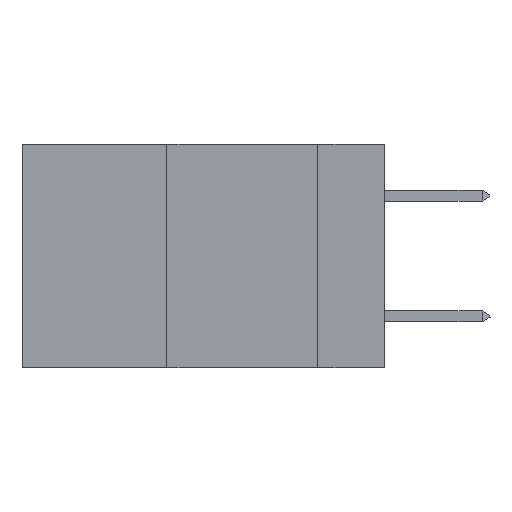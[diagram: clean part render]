
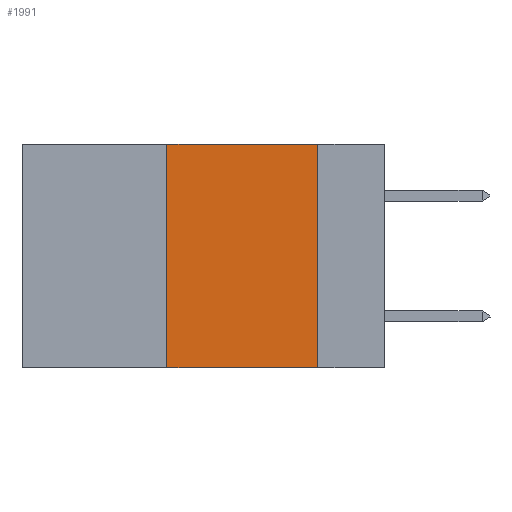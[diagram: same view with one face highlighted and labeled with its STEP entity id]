
A CAD part, left-side view. The second image highlights one B-rep face of the part: STEP entity #1991.
In plain terms, the highlighted planar face has unit normal (-1, 0, 0).
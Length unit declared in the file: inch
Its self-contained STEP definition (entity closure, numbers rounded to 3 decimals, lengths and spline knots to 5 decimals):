
#966 = ORIENTED_EDGE ( 'NONE', *, *, #12386, .F. ) ;
#1991 = ADVANCED_FACE ( 'NONE', ( #23413 ), #28684, .F. ) ;
#2405 = VECTOR ( 'NONE', #26414, 39.37008 ) ;
#3219 = LINE ( 'NONE', #21756, #11726 ) ;
#3683 = CARTESIAN_POINT ( 'NONE',  ( 0., 0.11, -0.37 ) ) ;
#4256 = AXIS2_PLACEMENT_3D ( 'NONE', #13226, #26502, #15324 ) ;
#4510 = LINE ( 'NONE', #13236, #2405 ) ;
#5833 = VECTOR ( 'NONE', #26191, 39.37008 ) ;
#6096 = VERTEX_POINT ( 'NONE', #9313 ) ;
#6454 = EDGE_LOOP ( 'NONE', ( #27809, #10366, #966, #25766 ) ) ;
#7420 = CARTESIAN_POINT ( 'NONE',  ( 0., 0.36, -0.37 ) ) ;
#9313 = CARTESIAN_POINT ( 'NONE',  ( 0., 0.36, 0. ) ) ;
#10366 = ORIENTED_EDGE ( 'NONE', *, *, #11468, .F. ) ;
#11468 = EDGE_CURVE ( 'NONE', #6096, #14197, #4510, .T. ) ;
#11726 = VECTOR ( 'NONE', #21947, 39.37008 ) ;
#11826 = VECTOR ( 'NONE', #12372, 39.37008 ) ;
#12372 = DIRECTION ( 'NONE',  ( 0., -1., 0. ) ) ;
#12386 = EDGE_CURVE ( 'NONE', #21610, #6096, #17920, .T. ) ;
#13226 = CARTESIAN_POINT ( 'NONE',  ( 0., 0.6, 0. ) ) ;
#13236 = CARTESIAN_POINT ( 'NONE',  ( 0., 0.6, 0. ) ) ;
#14197 = VERTEX_POINT ( 'NONE', #23990 ) ;
#15324 = DIRECTION ( 'NONE',  ( 0., 0., -1. ) ) ;
#17920 = LINE ( 'NONE', #26490, #5833 ) ;
#17947 = EDGE_CURVE ( 'NONE', #14197, #18339, #3219, .T. ) ;
#18339 = VERTEX_POINT ( 'NONE', #3683 ) ;
#18994 = CARTESIAN_POINT ( 'NONE',  ( 0., 0.6, -0.37 ) ) ;
#21610 = VERTEX_POINT ( 'NONE', #7420 ) ;
#21708 = LINE ( 'NONE', #18994, #11826 ) ;
#21756 = CARTESIAN_POINT ( 'NONE',  ( 0., 0.11, 0. ) ) ;
#21947 = DIRECTION ( 'NONE',  ( 0., 0., -1. ) ) ;
#23413 = FACE_OUTER_BOUND ( 'NONE', #6454, .T. ) ;
#23990 = CARTESIAN_POINT ( 'NONE',  ( 0., 0.11, 0. ) ) ;
#24893 = EDGE_CURVE ( 'NONE', #21610, #18339, #21708, .T. ) ;
#25766 = ORIENTED_EDGE ( 'NONE', *, *, #24893, .T. ) ;
#26191 = DIRECTION ( 'NONE',  ( 0., 0., 1. ) ) ;
#26414 = DIRECTION ( 'NONE',  ( 0., -1., 0. ) ) ;
#26490 = CARTESIAN_POINT ( 'NONE',  ( 0., 0.36, 0. ) ) ;
#26502 = DIRECTION ( 'NONE',  ( 1., 0., 0. ) ) ;
#27809 = ORIENTED_EDGE ( 'NONE', *, *, #17947, .F. ) ;
#28684 = PLANE ( 'NONE',  #4256 ) ;
